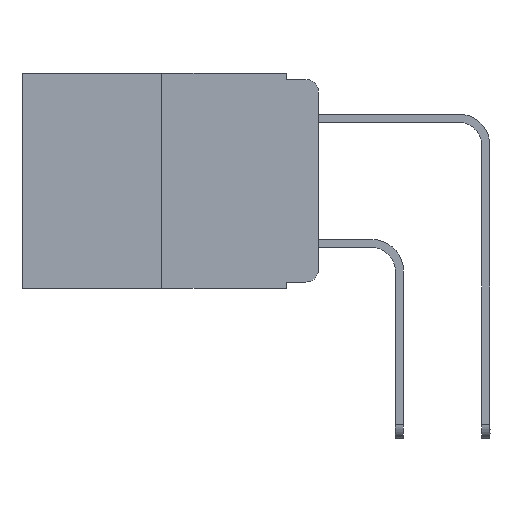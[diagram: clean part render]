
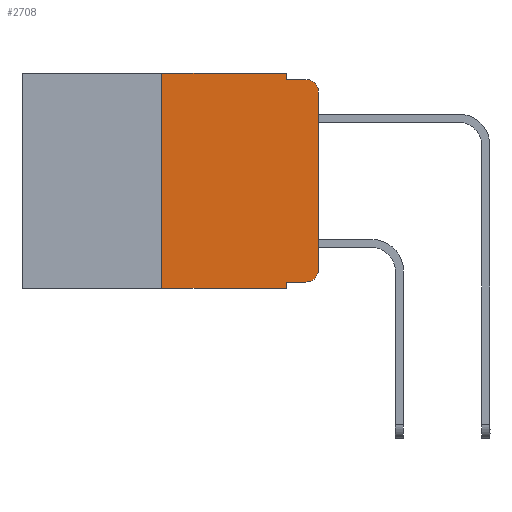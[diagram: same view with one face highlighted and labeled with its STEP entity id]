
A CAD part, left-side view. The second image highlights one B-rep face of the part: STEP entity #2708.
In plain terms, the highlighted planar face has unit normal (-1, 0, 0).
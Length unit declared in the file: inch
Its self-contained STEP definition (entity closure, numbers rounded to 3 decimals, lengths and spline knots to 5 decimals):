
#90 = EDGE_CURVE ( 'NONE', #13884, #7422, #4837, .T. ) ;
#99 = VECTOR ( 'NONE', #13005, 39.37008 ) ;
#405 = CARTESIAN_POINT ( 'NONE',  ( 0., 0.051, -0.343 ) ) ;
#424 = EDGE_CURVE ( 'NONE', #3310, #10578, #5649, .T. ) ;
#497 = DIRECTION ( 'NONE',  ( 0., -1., 0. ) ) ;
#600 = CARTESIAN_POINT ( 'NONE',  ( 0., 0.473, -0.343 ) ) ;
#779 = DIRECTION ( 'NONE',  ( 0., -1., 0. ) ) ;
#840 = CIRCLE ( 'NONE', #6793, 0.02 ) ;
#941 = LINE ( 'NONE', #7240, #1071 ) ;
#1067 = ORIENTED_EDGE ( 'NONE', *, *, #424, .F. ) ;
#1071 = VECTOR ( 'NONE', #11378, 39.37008 ) ;
#1878 = AXIS2_PLACEMENT_3D ( 'NONE', #14136, #9314, #12184 ) ;
#2289 = VERTEX_POINT ( 'NONE', #7570 ) ;
#2575 = ORIENTED_EDGE ( 'NONE', *, *, #17330, .T. ) ;
#2708 = ADVANCED_FACE ( 'NONE', ( #3008 ), #13831, .F. ) ;
#3008 = FACE_OUTER_BOUND ( 'NONE', #20102, .T. ) ;
#3015 = EDGE_CURVE ( 'NONE', #3310, #7422, #5044, .T. ) ;
#3081 = EDGE_CURVE ( 'NONE', #16707, #8538, #840, .T. ) ;
#3310 = VERTEX_POINT ( 'NONE', #13209 ) ;
#3435 = VERTEX_POINT ( 'NONE', #5379 ) ;
#3999 = VECTOR ( 'NONE', #15280, 39.37008 ) ;
#4014 = CARTESIAN_POINT ( 'NONE',  ( 0., 0.25, 0. ) ) ;
#4410 = DIRECTION ( 'NONE',  ( 0., 0., -1. ) ) ;
#4597 = AXIS2_PLACEMENT_3D ( 'NONE', #9356, #4803, #11098 ) ;
#4757 = CARTESIAN_POINT ( 'NONE',  ( 0., 0.051, -0.333 ) ) ;
#4803 = DIRECTION ( 'NONE',  ( -1., 0., 0. ) ) ;
#4837 = LINE ( 'NONE', #6178, #12981 ) ;
#4930 = VECTOR ( 'NONE', #779, 39.37008 ) ;
#5044 = LINE ( 'NONE', #600, #6109 ) ;
#5239 = CARTESIAN_POINT ( 'NONE',  ( 0., 0.02, -0.333 ) ) ;
#5379 = CARTESIAN_POINT ( 'NONE',  ( 0., 0.051, -0.01 ) ) ;
#5426 = ORIENTED_EDGE ( 'NONE', *, *, #8742, .T. ) ;
#5470 = EDGE_CURVE ( 'NONE', #17750, #2289, #18107, .T. ) ;
#5649 = LINE ( 'NONE', #4014, #15283 ) ;
#6109 = VECTOR ( 'NONE', #497, 39.37008 ) ;
#6149 = ORIENTED_EDGE ( 'NONE', *, *, #10811, .F. ) ;
#6178 = CARTESIAN_POINT ( 'NONE',  ( 0., 0.051, 0. ) ) ;
#6333 = EDGE_CURVE ( 'NONE', #10578, #11893, #8259, .T. ) ;
#6765 = EDGE_CURVE ( 'NONE', #3435, #2289, #6777, .T. ) ;
#6777 = LINE ( 'NONE', #19568, #4930 ) ;
#6793 = AXIS2_PLACEMENT_3D ( 'NONE', #19288, #11449, #11227 ) ;
#7240 = CARTESIAN_POINT ( 'NONE',  ( 0., 0., 0. ) ) ;
#7422 = VERTEX_POINT ( 'NONE', #405 ) ;
#7570 = CARTESIAN_POINT ( 'NONE',  ( 0., 0.02, -0.01 ) ) ;
#7623 = CARTESIAN_POINT ( 'NONE',  ( 0., 0., -0.03 ) ) ;
#7921 = DIRECTION ( 'NONE',  ( 0., 0., -1. ) ) ;
#8259 = LINE ( 'NONE', #14446, #99 ) ;
#8538 = VERTEX_POINT ( 'NONE', #17806 ) ;
#8742 = EDGE_CURVE ( 'NONE', #13884, #16707, #18771, .T. ) ;
#9253 = CARTESIAN_POINT ( 'NONE',  ( 0., 0.051, 0. ) ) ;
#9314 = DIRECTION ( 'NONE',  ( 1., 0., 0. ) ) ;
#9356 = CARTESIAN_POINT ( 'NONE',  ( 0., 0.02, -0.03 ) ) ;
#9663 = VECTOR ( 'NONE', #4410, 39.37008 ) ;
#10578 = VERTEX_POINT ( 'NONE', #13577 ) ;
#10811 = EDGE_CURVE ( 'NONE', #11893, #3435, #20180, .T. ) ;
#11098 = DIRECTION ( 'NONE',  ( 0., 0., -1. ) ) ;
#11227 = DIRECTION ( 'NONE',  ( 0., 0., -1. ) ) ;
#11330 = ORIENTED_EDGE ( 'NONE', *, *, #3015, .T. ) ;
#11378 = DIRECTION ( 'NONE',  ( 0., 0., 1. ) ) ;
#11449 = DIRECTION ( 'NONE',  ( -1., 0., 0. ) ) ;
#11893 = VERTEX_POINT ( 'NONE', #18028 ) ;
#12184 = DIRECTION ( 'NONE',  ( 0., 0., -1. ) ) ;
#12505 = ORIENTED_EDGE ( 'NONE', *, *, #6333, .F. ) ;
#12568 = ORIENTED_EDGE ( 'NONE', *, *, #5470, .T. ) ;
#12595 = CARTESIAN_POINT ( 'NONE',  ( 0., 0.051, -0.333 ) ) ;
#12981 = VECTOR ( 'NONE', #7921, 39.37008 ) ;
#13005 = DIRECTION ( 'NONE',  ( 0., -1., 0. ) ) ;
#13209 = CARTESIAN_POINT ( 'NONE',  ( 0., 0.25, -0.343 ) ) ;
#13577 = CARTESIAN_POINT ( 'NONE',  ( 0., 0.25, 0. ) ) ;
#13831 = PLANE ( 'NONE',  #1878 ) ;
#13884 = VERTEX_POINT ( 'NONE', #12595 ) ;
#14136 = CARTESIAN_POINT ( 'NONE',  ( 0., 0.473, 0. ) ) ;
#14446 = CARTESIAN_POINT ( 'NONE',  ( 0., 0.473, 0. ) ) ;
#15280 = DIRECTION ( 'NONE',  ( 0., -1., 0. ) ) ;
#15283 = VECTOR ( 'NONE', #16889, 39.37008 ) ;
#15823 = ORIENTED_EDGE ( 'NONE', *, *, #3081, .T. ) ;
#16684 = ORIENTED_EDGE ( 'NONE', *, *, #6765, .F. ) ;
#16707 = VERTEX_POINT ( 'NONE', #5239 ) ;
#16889 = DIRECTION ( 'NONE',  ( 0., 0., 1. ) ) ;
#17330 = EDGE_CURVE ( 'NONE', #8538, #17750, #941, .T. ) ;
#17750 = VERTEX_POINT ( 'NONE', #7623 ) ;
#17806 = CARTESIAN_POINT ( 'NONE',  ( 0., 0., -0.313 ) ) ;
#18028 = CARTESIAN_POINT ( 'NONE',  ( 0., 0.051, 0. ) ) ;
#18107 = CIRCLE ( 'NONE', #4597, 0.02 ) ;
#18771 = LINE ( 'NONE', #4757, #3999 ) ;
#19288 = CARTESIAN_POINT ( 'NONE',  ( 0., 0.02, -0.313 ) ) ;
#19568 = CARTESIAN_POINT ( 'NONE',  ( 0., 0.051, -0.01 ) ) ;
#19978 = ORIENTED_EDGE ( 'NONE', *, *, #90, .F. ) ;
#20102 = EDGE_LOOP ( 'NONE', ( #2575, #12568, #16684, #6149, #12505, #1067, #11330, #19978, #5426, #15823 ) ) ;
#20180 = LINE ( 'NONE', #9253, #9663 ) ;
